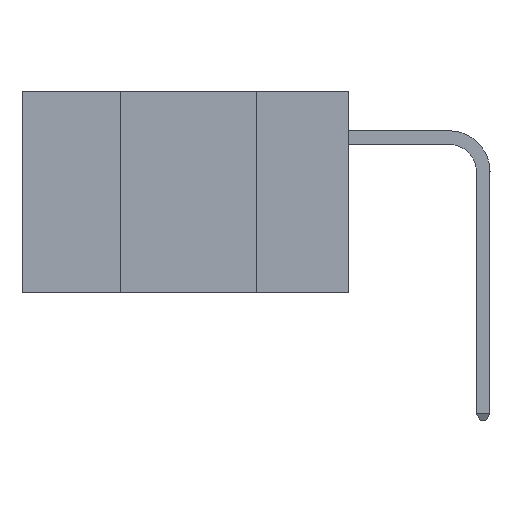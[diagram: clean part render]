
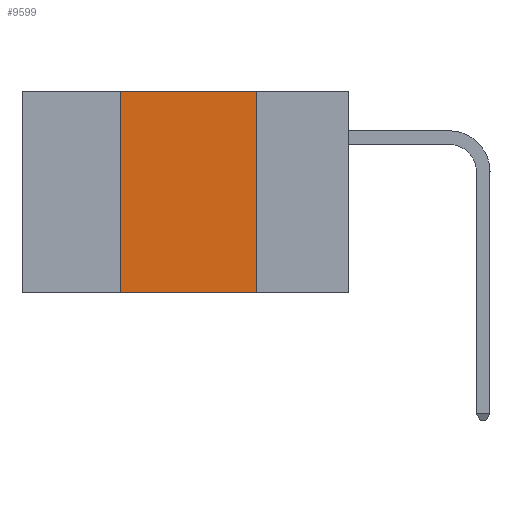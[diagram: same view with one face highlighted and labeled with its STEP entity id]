
A CAD part, left-side view. The second image highlights one B-rep face of the part: STEP entity #9599.
In plain terms, the highlighted planar face has unit normal (-1, 0, 0).
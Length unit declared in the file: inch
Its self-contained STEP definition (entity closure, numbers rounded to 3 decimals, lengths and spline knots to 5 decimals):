
#181 = CARTESIAN_POINT ( 'NONE',  ( 0., 0.6, 0. ) ) ;
#984 = ORIENTED_EDGE ( 'NONE', *, *, #6722, .F. ) ;
#1654 = VECTOR ( 'NONE', #6336, 39.37008 ) ;
#2641 = EDGE_CURVE ( 'NONE', #7058, #4623, #2928, .T. ) ;
#2885 = EDGE_LOOP ( 'NONE', ( #25251, #984, #7386, #19621 ) ) ;
#2928 = LINE ( 'NONE', #20648, #24154 ) ;
#3367 = AXIS2_PLACEMENT_3D ( 'NONE', #181, #4656, #18996 ) ;
#3444 = FACE_OUTER_BOUND ( 'NONE', #2885, .T. ) ;
#3592 = VECTOR ( 'NONE', #19789, 39.37008 ) ;
#4215 = CARTESIAN_POINT ( 'NONE',  ( 0., 0.6, 0. ) ) ;
#4623 = VERTEX_POINT ( 'NONE', #8456 ) ;
#4656 = DIRECTION ( 'NONE',  ( 1., 0., 0. ) ) ;
#6282 = DIRECTION ( 'NONE',  ( 0., 0., -1. ) ) ;
#6336 = DIRECTION ( 'NONE',  ( 0., -1., 0. ) ) ;
#6640 = PLANE ( 'NONE',  #3367 ) ;
#6722 = EDGE_CURVE ( 'NONE', #4623, #10170, #7381, .T. ) ;
#7058 = VERTEX_POINT ( 'NONE', #11623 ) ;
#7381 = LINE ( 'NONE', #4215, #1654 ) ;
#7386 = ORIENTED_EDGE ( 'NONE', *, *, #2641, .F. ) ;
#8456 = CARTESIAN_POINT ( 'NONE',  ( 0., 0.42, 0. ) ) ;
#8732 = CARTESIAN_POINT ( 'NONE',  ( 0., 0.17, 0. ) ) ;
#8810 = VERTEX_POINT ( 'NONE', #18426 ) ;
#9096 = LINE ( 'NONE', #15743, #3592 ) ;
#9599 = ADVANCED_FACE ( 'NONE', ( #3444 ), #6640, .F. ) ;
#9996 = EDGE_CURVE ( 'NONE', #10170, #8810, #15142, .T. ) ;
#10170 = VERTEX_POINT ( 'NONE', #8732 ) ;
#11623 = CARTESIAN_POINT ( 'NONE',  ( 0., 0.42, -0.37 ) ) ;
#15142 = LINE ( 'NONE', #16518, #19863 ) ;
#15743 = CARTESIAN_POINT ( 'NONE',  ( 0., 0.6, -0.37 ) ) ;
#16518 = CARTESIAN_POINT ( 'NONE',  ( 0., 0.17, 0. ) ) ;
#16680 = DIRECTION ( 'NONE',  ( 0., 0., 1. ) ) ;
#18426 = CARTESIAN_POINT ( 'NONE',  ( 0., 0.17, -0.37 ) ) ;
#18996 = DIRECTION ( 'NONE',  ( 0., 0., -1. ) ) ;
#19621 = ORIENTED_EDGE ( 'NONE', *, *, #23823, .T. ) ;
#19789 = DIRECTION ( 'NONE',  ( 0., -1., 0. ) ) ;
#19863 = VECTOR ( 'NONE', #6282, 39.37008 ) ;
#20648 = CARTESIAN_POINT ( 'NONE',  ( 0., 0.42, 0. ) ) ;
#23823 = EDGE_CURVE ( 'NONE', #7058, #8810, #9096, .T. ) ;
#24154 = VECTOR ( 'NONE', #16680, 39.37008 ) ;
#25251 = ORIENTED_EDGE ( 'NONE', *, *, #9996, .F. ) ;
